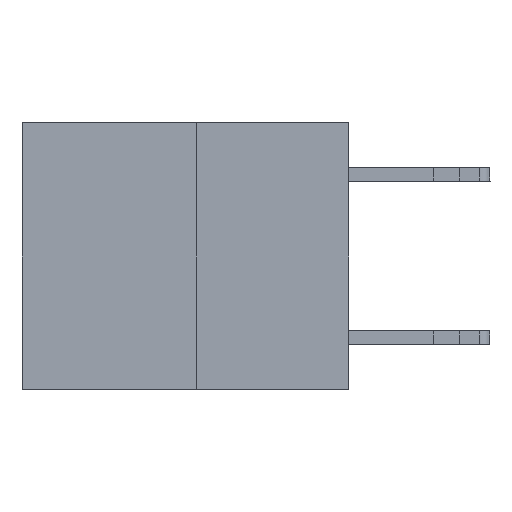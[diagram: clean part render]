
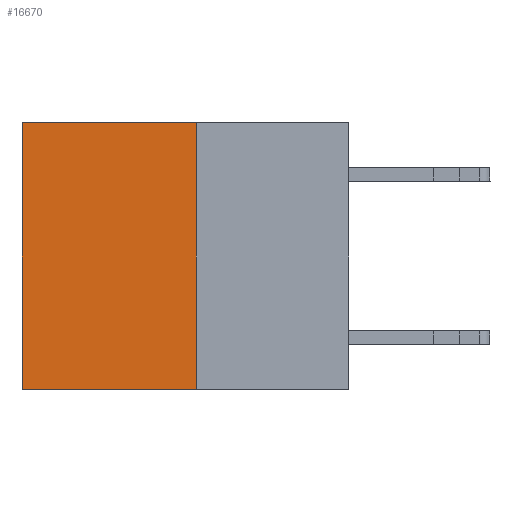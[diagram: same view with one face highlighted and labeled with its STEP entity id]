
A CAD part, left-side view. The second image highlights one B-rep face of the part: STEP entity #16670.
In plain terms, the highlighted planar face has unit normal (-1, 0, 0).
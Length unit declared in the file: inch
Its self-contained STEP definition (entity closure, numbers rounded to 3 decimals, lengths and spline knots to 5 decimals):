
#172 = ORIENTED_EDGE ( 'NONE', *, *, #12734, .F. ) ;
#317 = EDGE_CURVE ( 'NONE', #21556, #5782, #3459, .T. ) ;
#565 = FACE_OUTER_BOUND ( 'NONE', #8928, .T. ) ;
#998 = EDGE_CURVE ( 'NONE', #21556, #16503, #16231, .T. ) ;
#1200 = EDGE_CURVE ( 'NONE', #5782, #1637, #8124, .T. ) ;
#1637 = VERTEX_POINT ( 'NONE', #14635 ) ;
#2202 = VECTOR ( 'NONE', #15866, 39.37008 ) ;
#2706 = PLANE ( 'NONE',  #4004 ) ;
#2840 = VECTOR ( 'NONE', #6330, 39.37008 ) ;
#3459 = LINE ( 'NONE', #25685, #2202 ) ;
#4004 = AXIS2_PLACEMENT_3D ( 'NONE', #21028, #8799, #17006 ) ;
#4496 = ORIENTED_EDGE ( 'NONE', *, *, #998, .F. ) ;
#5782 = VERTEX_POINT ( 'NONE', #20853 ) ;
#6330 = DIRECTION ( 'NONE',  ( 0., 0., -1. ) ) ;
#7566 = DIRECTION ( 'NONE',  ( 0., 0., -1. ) ) ;
#8124 = LINE ( 'NONE', #12405, #2840 ) ;
#8799 = DIRECTION ( 'NONE',  ( 1., 0., 0. ) ) ;
#8928 = EDGE_LOOP ( 'NONE', ( #18479, #172, #4496, #9483 ) ) ;
#9483 = ORIENTED_EDGE ( 'NONE', *, *, #317, .T. ) ;
#9717 = CARTESIAN_POINT ( 'NONE',  ( 0.3165, 0.28, -0.49 ) ) ;
#10446 = LINE ( 'NONE', #23078, #19176 ) ;
#12405 = CARTESIAN_POINT ( 'NONE',  ( 0.3165, 0.6, -0.49 ) ) ;
#12734 = EDGE_CURVE ( 'NONE', #16503, #1637, #10446, .T. ) ;
#13504 = CARTESIAN_POINT ( 'NONE',  ( 0.3165, 0.28, 0. ) ) ;
#14635 = CARTESIAN_POINT ( 'NONE',  ( 0.3165, 0.6, -0.49 ) ) ;
#15350 = VECTOR ( 'NONE', #7566, 39.37008 ) ;
#15866 = DIRECTION ( 'NONE',  ( 0., 1., 0. ) ) ;
#16167 = CARTESIAN_POINT ( 'NONE',  ( 0.3165, 0.28, -0.49 ) ) ;
#16231 = LINE ( 'NONE', #9717, #15350 ) ;
#16503 = VERTEX_POINT ( 'NONE', #16167 ) ;
#16670 = ADVANCED_FACE ( 'NONE', ( #565 ), #2706, .F. ) ;
#17006 = DIRECTION ( 'NONE',  ( 0., 0., -1. ) ) ;
#18479 = ORIENTED_EDGE ( 'NONE', *, *, #1200, .T. ) ;
#19176 = VECTOR ( 'NONE', #23165, 39.37008 ) ;
#20853 = CARTESIAN_POINT ( 'NONE',  ( 0.3165, 0.6, 0. ) ) ;
#21028 = CARTESIAN_POINT ( 'NONE',  ( 0.3165, 0.28, -0.49 ) ) ;
#21556 = VERTEX_POINT ( 'NONE', #13504 ) ;
#23078 = CARTESIAN_POINT ( 'NONE',  ( 0.3165, 0.28, -0.49 ) ) ;
#23165 = DIRECTION ( 'NONE',  ( 0., 1., 0. ) ) ;
#25685 = CARTESIAN_POINT ( 'NONE',  ( 0.3165, 0.28, 0. ) ) ;
